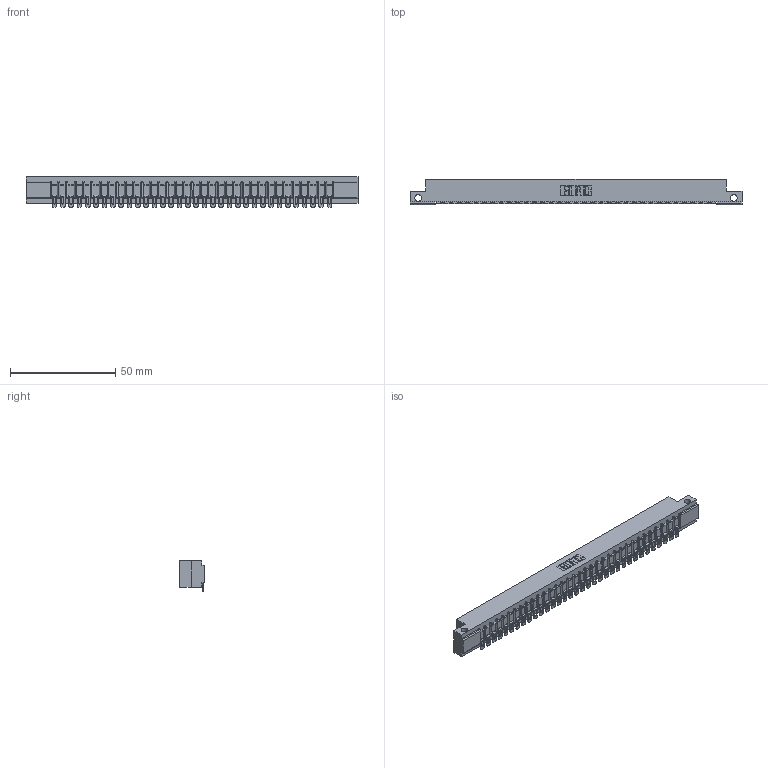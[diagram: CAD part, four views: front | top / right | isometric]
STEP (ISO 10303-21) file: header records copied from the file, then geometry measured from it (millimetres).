
FILE_DESCRIPTION (( 'STEP AP203' ), '1' );
FILE_NAME ('357-034-554-112.STEP', '2019-09-17T05:37:31', ( '' ), ( '' ), 'SwSTEP 2.0', 'SolidWorks 2016', '' );
FILE_SCHEMA (( 'CONFIG_CONTROL_DESIGN' ));
Length unit declared in the file: inch
Products named in the file (3): 307-290-002_554; 307 Part_.128 Dia Side Mounting Holes; 357-034-554-112
Assembly tree (35 placements, depth 2):
  357-034-554-112
    307 Part_.128 Dia Side Mounting Holes
    307-290-002_554  x34
Bounding box: 157.73 x 12.01 x 14.52 mm (x, y, z)
Volume: 16690 mm3; surface area: 20930.2 mm2
Topology: 35 solids, 35 shells, 2907 faces, 8925 edges, 5854 vertices
Faces by surface type: plane 1634, cylinder 1203, sphere 70
Entity records: 31101 total; most frequent: CARTESIAN_POINT 5246, ORIENTED_EDGE 5236, DIRECTION 5106, EDGE_CURVE 2618, LINE 1994, VECTOR 1994, VERTEX_POINT 1696, AXIS2_PLACEMENT_3D 1556
